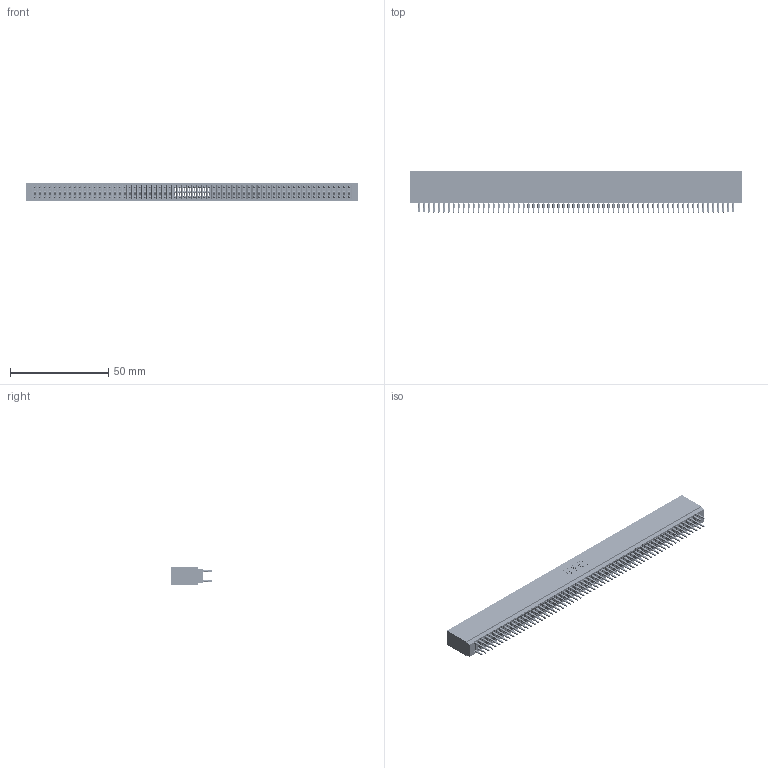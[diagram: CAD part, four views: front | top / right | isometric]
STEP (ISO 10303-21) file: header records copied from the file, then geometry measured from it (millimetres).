
FILE_DESCRIPTION (( 'STEP AP203' ), '1' );
FILE_NAME ('745-128-560-201.STEP', '2020-09-14T19:01:45', ( '' ), ( '' ), 'SwSTEP 2.0', 'SolidWorks 2020', '' );
FILE_SCHEMA (( 'CONFIG_CONTROL_DESIGN' ));
Length unit declared in the file: inch
Products named in the file (3): 745-292-001_560; 745 Part_Insulator Option - 01; 745-128-560-201
Assembly tree (129 placements, depth 2):
  745-128-560-201
    745 Part_Insulator Option - 01
    745-292-001_560  x128
Bounding box: 169.16 x 21.22 x 8.89 mm (x, y, z)
Volume: 15575.3 mm3; surface area: 34191.4 mm2
Topology: 129 solids, 129 shells, 12703 faces, 34754 edges, 22060 vertices
Faces by surface type: plane 6583, cylinder 2792, bspline 2560, torus 768
Entity records: 105071 total; most frequent: CARTESIAN_POINT 18721, ORIENTED_EDGE 18200, DIRECTION 15884, EDGE_CURVE 9100, LINE 8526, VECTOR 8526, VERTEX_POINT 5804, AXIS2_PLACEMENT_3D 3679
